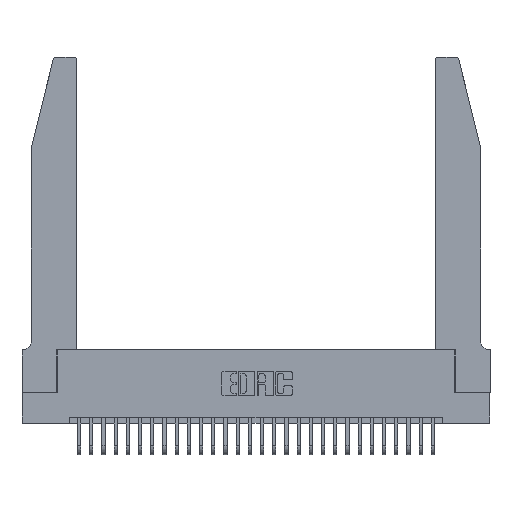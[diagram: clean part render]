
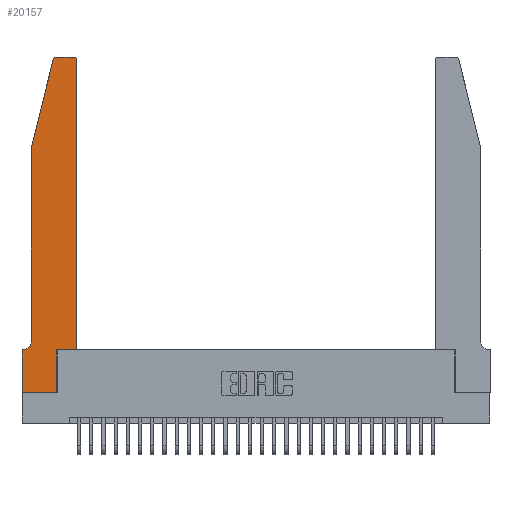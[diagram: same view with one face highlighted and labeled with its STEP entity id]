
A CAD part, top view. The second image highlights one B-rep face of the part: STEP entity #20157.
In plain terms, the highlighted planar face has unit normal (0, 0, 1).
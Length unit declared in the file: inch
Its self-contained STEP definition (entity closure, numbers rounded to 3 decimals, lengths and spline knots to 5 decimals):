
#940 = CARTESIAN_POINT ( 'NONE',  ( 0.2605, 2.75, 0.37 ) ) ;
#1263 = DIRECTION ( 'NONE',  ( 1., 0., 0. ) ) ;
#1268 = DIRECTION ( 'NONE',  ( 0., 1., 0. ) ) ;
#2238 = VERTEX_POINT ( 'NONE', #3056 ) ;
#2291 = LINE ( 'NONE', #21820, #19456 ) ;
#2331 = ORIENTED_EDGE ( 'NONE', *, *, #25683, .T. ) ;
#2783 = DIRECTION ( 'NONE',  ( -1., 0., 0. ) ) ;
#3056 = CARTESIAN_POINT ( 'NONE',  ( 0.2865, 0.35, 0.37 ) ) ;
#3163 = VERTEX_POINT ( 'NONE', #26785 ) ;
#3412 = CARTESIAN_POINT ( 'NONE',  ( 0.4505, 0.35, 0.37 ) ) ;
#3720 = CARTESIAN_POINT ( 'NONE',  ( 0.4505, 0.35, 0.37 ) ) ;
#4291 = AXIS2_PLACEMENT_3D ( 'NONE', #10753, #27781, #28103 ) ;
#4453 = DIRECTION ( 'NONE',  ( -1., 0., 0. ) ) ;
#4551 = LINE ( 'NONE', #18596, #22109 ) ;
#4733 = CARTESIAN_POINT ( 'NONE',  ( 0.0755, 2., 0.37 ) ) ;
#4749 = ORIENTED_EDGE ( 'NONE', *, *, #15123, .T. ) ;
#5053 = LINE ( 'NONE', #940, #20702 ) ;
#5074 = EDGE_CURVE ( 'NONE', #5519, #19015, #5053, .T. ) ;
#5519 = VERTEX_POINT ( 'NONE', #21886 ) ;
#5639 = CARTESIAN_POINT ( 'NONE',  ( 0.4505, 2.72, 0.37 ) ) ;
#5957 = VERTEX_POINT ( 'NONE', #20046 ) ;
#5958 = VECTOR ( 'NONE', #10534, 39.37008 ) ;
#6051 = PLANE ( 'NONE',  #4291 ) ;
#6208 = AXIS2_PLACEMENT_3D ( 'NONE', #23433, #18652, #8834 ) ;
#6310 = DIRECTION ( 'NONE',  ( 0., -1., 0. ) ) ;
#7067 = EDGE_CURVE ( 'NONE', #5957, #24082, #4551, .T. ) ;
#7128 = DIRECTION ( 'NONE',  ( 1., 0., 0. ) ) ;
#8834 = DIRECTION ( 'NONE',  ( 1., 0., 0. ) ) ;
#8954 = CARTESIAN_POINT ( 'NONE',  ( 0.0755, 0.42, 0.37 ) ) ;
#9623 = FACE_OUTER_BOUND ( 'NONE', #24933, .T. ) ;
#9654 = DIRECTION ( 'NONE',  ( -0.239, -0.971, 0. ) ) ;
#9729 = VECTOR ( 'NONE', #4453, 39.37008 ) ;
#10534 = DIRECTION ( 'NONE',  ( 0., 1., 0. ) ) ;
#10753 = CARTESIAN_POINT ( 'NONE',  ( 0., 0.35, 0.37 ) ) ;
#11051 = EDGE_CURVE ( 'NONE', #29878, #12506, #11326, .T. ) ;
#11205 = CARTESIAN_POINT ( 'NONE',  ( 0., 0., 0.37 ) ) ;
#11326 = LINE ( 'NONE', #14829, #29283 ) ;
#11624 = EDGE_CURVE ( 'NONE', #12506, #3163, #2291, .T. ) ;
#12082 = VECTOR ( 'NONE', #1268, 39.37008 ) ;
#12290 = VERTEX_POINT ( 'NONE', #5639 ) ;
#12374 = ORIENTED_EDGE ( 'NONE', *, *, #27741, .T. ) ;
#12448 = VERTEX_POINT ( 'NONE', #30363 ) ;
#12506 = VERTEX_POINT ( 'NONE', #11205 ) ;
#12508 = CARTESIAN_POINT ( 'NONE',  ( 0.0055, 0.42, 0.37 ) ) ;
#13659 = LINE ( 'NONE', #4733, #20872 ) ;
#13665 = LINE ( 'NONE', #3720, #17462 ) ;
#13942 = AXIS2_PLACEMENT_3D ( 'NONE', #18877, #19296, #7128 ) ;
#14447 = EDGE_CURVE ( 'NONE', #3163, #2238, #23879, .T. ) ;
#14829 = CARTESIAN_POINT ( 'NONE',  ( 0., 0., 0.37 ) ) ;
#15123 = EDGE_CURVE ( 'NONE', #20788, #29878, #18520, .T. ) ;
#15640 = CARTESIAN_POINT ( 'NONE',  ( 0.0055, 0.35, 0.37 ) ) ;
#17181 = EDGE_CURVE ( 'NONE', #12290, #5519, #17228, .T. ) ;
#17228 = CIRCLE ( 'NONE', #6208, 0.03 ) ;
#17405 = DIRECTION ( 'NONE',  ( 0., 0., -1. ) ) ;
#17462 = VECTOR ( 'NONE', #1263, 39.37008 ) ;
#18215 = CARTESIAN_POINT ( 'NONE',  ( 0.2865, 0.35, 0.37 ) ) ;
#18337 = DIRECTION ( 'NONE',  ( -1., 0., 0. ) ) ;
#18520 = LINE ( 'NONE', #26233, #9729 ) ;
#18596 = CARTESIAN_POINT ( 'NONE',  ( 0.0755, 2., 0.37 ) ) ;
#18652 = DIRECTION ( 'NONE',  ( 0., 0., 1. ) ) ;
#18877 = CARTESIAN_POINT ( 'NONE',  ( 0.284, 2.72, 0.37 ) ) ;
#18940 = ORIENTED_EDGE ( 'NONE', *, *, #11624, .T. ) ;
#19015 = VERTEX_POINT ( 'NONE', #22895 ) ;
#19296 = DIRECTION ( 'NONE',  ( 0., 0., 1. ) ) ;
#19445 = ORIENTED_EDGE ( 'NONE', *, *, #11051, .T. ) ;
#19456 = VECTOR ( 'NONE', #24704, 39.37008 ) ;
#19827 = ORIENTED_EDGE ( 'NONE', *, *, #14447, .T. ) ;
#20012 = ORIENTED_EDGE ( 'NONE', *, *, #23032, .T. ) ;
#20046 = CARTESIAN_POINT ( 'NONE',  ( 0.0755, 2., 0.37 ) ) ;
#20157 = ADVANCED_FACE ( 'NONE', ( #9623 ), #6051, .T. ) ;
#20702 = VECTOR ( 'NONE', #18337, 39.37008 ) ;
#20788 = VERTEX_POINT ( 'NONE', #15640 ) ;
#20872 = VECTOR ( 'NONE', #9654, 39.37008 ) ;
#21008 = ORIENTED_EDGE ( 'NONE', *, *, #5074, .T. ) ;
#21791 = EDGE_CURVE ( 'NONE', #19015, #12448, #24022, .T. ) ;
#21820 = CARTESIAN_POINT ( 'NONE',  ( 0., 0., 0.37 ) ) ;
#21886 = CARTESIAN_POINT ( 'NONE',  ( 0.4205, 2.75, 0.37 ) ) ;
#22109 = VECTOR ( 'NONE', #6310, 39.37008 ) ;
#22344 = ORIENTED_EDGE ( 'NONE', *, *, #26250, .T. ) ;
#22351 = AXIS2_PLACEMENT_3D ( 'NONE', #12508, #17405, #2783 ) ;
#22895 = CARTESIAN_POINT ( 'NONE',  ( 0.284, 2.75, 0.37 ) ) ;
#23032 = EDGE_CURVE ( 'NONE', #12448, #5957, #13659, .T. ) ;
#23433 = CARTESIAN_POINT ( 'NONE',  ( 0.4205, 2.72, 0.37 ) ) ;
#23879 = LINE ( 'NONE', #18215, #5958 ) ;
#23938 = VERTEX_POINT ( 'NONE', #3412 ) ;
#24022 = CIRCLE ( 'NONE', #13942, 0.03 ) ;
#24082 = VERTEX_POINT ( 'NONE', #8954 ) ;
#24309 = CARTESIAN_POINT ( 'NONE',  ( 0., 0.35, 0.37 ) ) ;
#24704 = DIRECTION ( 'NONE',  ( 1., 0., 0. ) ) ;
#24864 = ORIENTED_EDGE ( 'NONE', *, *, #7067, .T. ) ;
#24933 = EDGE_LOOP ( 'NONE', ( #21008, #28220, #20012, #24864, #2331, #4749, #19445, #18940, #19827, #22344, #12374, #31341 ) ) ;
#25524 = CIRCLE ( 'NONE', #22351, 0.07 ) ;
#25683 = EDGE_CURVE ( 'NONE', #24082, #20788, #25524, .T. ) ;
#26233 = CARTESIAN_POINT ( 'NONE',  ( 0.0755, 0.35, 0.37 ) ) ;
#26250 = EDGE_CURVE ( 'NONE', #2238, #23938, #13665, .T. ) ;
#26785 = CARTESIAN_POINT ( 'NONE',  ( 0.2865, 0., 0.37 ) ) ;
#27344 = DIRECTION ( 'NONE',  ( 0., -1., 0. ) ) ;
#27741 = EDGE_CURVE ( 'NONE', #23938, #12290, #28446, .T. ) ;
#27781 = DIRECTION ( 'NONE',  ( 0., 0., 1. ) ) ;
#28103 = DIRECTION ( 'NONE',  ( 1., 0., 0. ) ) ;
#28220 = ORIENTED_EDGE ( 'NONE', *, *, #21791, .T. ) ;
#28446 = LINE ( 'NONE', #30366, #12082 ) ;
#29283 = VECTOR ( 'NONE', #27344, 39.37008 ) ;
#29878 = VERTEX_POINT ( 'NONE', #24309 ) ;
#30363 = CARTESIAN_POINT ( 'NONE',  ( 0.25487, 2.72718, 0.37 ) ) ;
#30366 = CARTESIAN_POINT ( 'NONE',  ( 0.4505, 0.35, 0.37 ) ) ;
#31341 = ORIENTED_EDGE ( 'NONE', *, *, #17181, .T. ) ;
